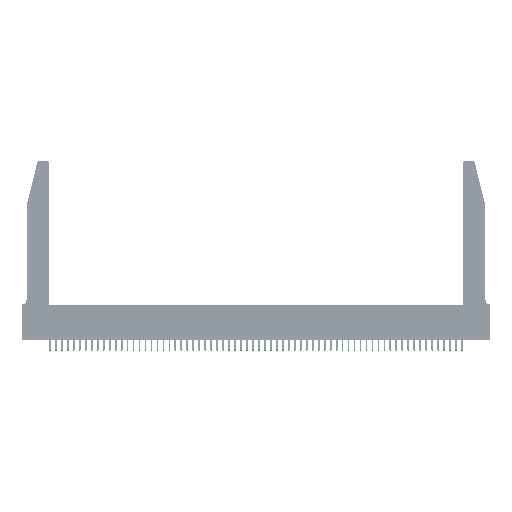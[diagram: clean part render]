
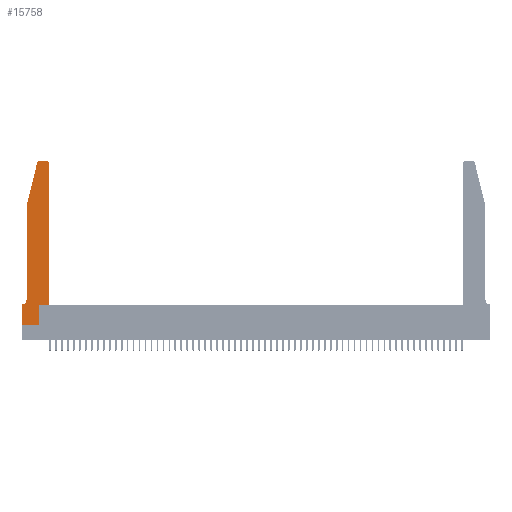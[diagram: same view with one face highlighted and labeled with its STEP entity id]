
A CAD part, top view. The second image highlights one B-rep face of the part: STEP entity #15758.
In plain terms, the highlighted planar face has unit normal (0, 0, 1).
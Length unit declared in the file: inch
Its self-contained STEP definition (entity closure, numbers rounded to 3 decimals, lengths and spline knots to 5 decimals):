
#101 = EDGE_CURVE ( 'NONE', #5792, #35913, #6823, .T. ) ;
#407 = VERTEX_POINT ( 'NONE', #45892 ) ;
#583 = LINE ( 'NONE', #42101, #45252 ) ;
#868 = VECTOR ( 'NONE', #31480, 39.37008 ) ;
#1223 = VERTEX_POINT ( 'NONE', #55118 ) ;
#1274 = EDGE_CURVE ( 'NONE', #35913, #38165, #583, .T. ) ;
#1558 = VECTOR ( 'NONE', #19152, 39.37008 ) ;
#2995 = DIRECTION ( 'NONE',  ( 0., 0., 1. ) ) ;
#3016 = DIRECTION ( 'NONE',  ( 0., 0., 1. ) ) ;
#3616 = CARTESIAN_POINT ( 'NONE',  ( 0., 0.35, 0.37 ) ) ;
#4064 = CARTESIAN_POINT ( 'NONE',  ( 0.0055, 0.35, 0.37 ) ) ;
#4310 = LINE ( 'NONE', #30976, #32062 ) ;
#5256 = EDGE_CURVE ( 'NONE', #407, #19347, #4310, .T. ) ;
#5743 = CARTESIAN_POINT ( 'NONE',  ( 0.4505, 0.35, 0.37 ) ) ;
#5792 = VERTEX_POINT ( 'NONE', #4064 ) ;
#6823 = LINE ( 'NONE', #33890, #46058 ) ;
#7276 = DIRECTION ( 'NONE',  ( 1., 0., 0. ) ) ;
#7305 = CARTESIAN_POINT ( 'NONE',  ( 0.0055, 0.42, 0.37 ) ) ;
#8950 = ORIENTED_EDGE ( 'NONE', *, *, #27693, .T. ) ;
#9331 = EDGE_LOOP ( 'NONE', ( #8950, #53865, #27278, #42686, #16671, #38875, #25576, #28283, #25086, #22221, #33995, #50335 ) ) ;
#10756 = EDGE_CURVE ( 'NONE', #41395, #11574, #15160, .T. ) ;
#11542 = DIRECTION ( 'NONE',  ( 0., 0., 1. ) ) ;
#11574 = VERTEX_POINT ( 'NONE', #22725 ) ;
#13098 = CARTESIAN_POINT ( 'NONE',  ( 0., 0., 0.37 ) ) ;
#15053 = CIRCLE ( 'NONE', #49882, 0.03 ) ;
#15160 = LINE ( 'NONE', #5743, #868 ) ;
#15224 = LINE ( 'NONE', #22927, #24682 ) ;
#15465 = AXIS2_PLACEMENT_3D ( 'NONE', #7305, #41891, #20745 ) ;
#15758 = ADVANCED_FACE ( 'NONE', ( #28016 ), #55628, .T. ) ;
#16457 = LINE ( 'NONE', #24059, #1558 ) ;
#16671 = ORIENTED_EDGE ( 'NONE', *, *, #50506, .T. ) ;
#17755 = CARTESIAN_POINT ( 'NONE',  ( 0.0755, 2., 0.37 ) ) ;
#19152 = DIRECTION ( 'NONE',  ( -1., 0., 0. ) ) ;
#19289 = EDGE_CURVE ( 'NONE', #19347, #20377, #46531, .T. ) ;
#19306 = DIRECTION ( 'NONE',  ( 0., 1., 0. ) ) ;
#19347 = VERTEX_POINT ( 'NONE', #17755 ) ;
#20377 = VERTEX_POINT ( 'NONE', #45859 ) ;
#20745 = DIRECTION ( 'NONE',  ( -1., 0., 0. ) ) ;
#20920 = LINE ( 'NONE', #24334, #43241 ) ;
#22221 = ORIENTED_EDGE ( 'NONE', *, *, #41916, .T. ) ;
#22725 = CARTESIAN_POINT ( 'NONE',  ( 0.4505, 2.72, 0.37 ) ) ;
#22927 = CARTESIAN_POINT ( 'NONE',  ( 0.2865, 0.35, 0.37 ) ) ;
#24059 = CARTESIAN_POINT ( 'NONE',  ( 0.2605, 2.75, 0.37 ) ) ;
#24334 = CARTESIAN_POINT ( 'NONE',  ( 0.4505, 0.35, 0.37 ) ) ;
#24589 = DIRECTION ( 'NONE',  ( 1., 0., 0. ) ) ;
#24682 = VECTOR ( 'NONE', #19306, 39.37008 ) ;
#25086 = ORIENTED_EDGE ( 'NONE', *, *, #36536, .T. ) ;
#25159 = CARTESIAN_POINT ( 'NONE',  ( 0.4505, 0.35, 0.37 ) ) ;
#25576 = ORIENTED_EDGE ( 'NONE', *, *, #1274, .T. ) ;
#25790 = DIRECTION ( 'NONE',  ( 1., 0., 0. ) ) ;
#26288 = AXIS2_PLACEMENT_3D ( 'NONE', #54805, #2995, #37589 ) ;
#26347 = LINE ( 'NONE', #13098, #45908 ) ;
#27278 = ORIENTED_EDGE ( 'NONE', *, *, #5256, .T. ) ;
#27693 = EDGE_CURVE ( 'NONE', #45223, #1223, #16457, .T. ) ;
#28016 = FACE_OUTER_BOUND ( 'NONE', #9331, .T. ) ;
#28283 = ORIENTED_EDGE ( 'NONE', *, *, #33462, .T. ) ;
#28641 = CARTESIAN_POINT ( 'NONE',  ( 0., 0., 0.37 ) ) ;
#30071 = CIRCLE ( 'NONE', #26288, 0.03 ) ;
#30976 = CARTESIAN_POINT ( 'NONE',  ( 0.0755, 2., 0.37 ) ) ;
#31480 = DIRECTION ( 'NONE',  ( 0., 1., 0. ) ) ;
#32062 = VECTOR ( 'NONE', #35497, 39.37008 ) ;
#33462 = EDGE_CURVE ( 'NONE', #38165, #39891, #26347, .T. ) ;
#33890 = CARTESIAN_POINT ( 'NONE',  ( 0.0755, 0.35, 0.37 ) ) ;
#33995 = ORIENTED_EDGE ( 'NONE', *, *, #10756, .T. ) ;
#34957 = CARTESIAN_POINT ( 'NONE',  ( 0.0755, 2., 0.37 ) ) ;
#35497 = DIRECTION ( 'NONE',  ( -0.239, -0.971, 0. ) ) ;
#35913 = VERTEX_POINT ( 'NONE', #53578 ) ;
#36536 = EDGE_CURVE ( 'NONE', #39891, #46829, #15224, .T. ) ;
#36779 = EDGE_CURVE ( 'NONE', #11574, #45223, #30071, .T. ) ;
#37046 = CARTESIAN_POINT ( 'NONE',  ( 0.284, 2.72, 0.37 ) ) ;
#37589 = DIRECTION ( 'NONE',  ( 1., 0., 0. ) ) ;
#37636 = CARTESIAN_POINT ( 'NONE',  ( 0.2865, 0.35, 0.37 ) ) ;
#37795 = EDGE_CURVE ( 'NONE', #1223, #407, #15053, .T. ) ;
#38165 = VERTEX_POINT ( 'NONE', #28641 ) ;
#38875 = ORIENTED_EDGE ( 'NONE', *, *, #101, .T. ) ;
#39060 = VECTOR ( 'NONE', #47475, 39.37008 ) ;
#39891 = VERTEX_POINT ( 'NONE', #47780 ) ;
#40790 = CARTESIAN_POINT ( 'NONE',  ( 0.4205, 2.75, 0.37 ) ) ;
#41395 = VERTEX_POINT ( 'NONE', #25159 ) ;
#41536 = DIRECTION ( 'NONE',  ( 0., -1., 0. ) ) ;
#41891 = DIRECTION ( 'NONE',  ( 0., 0., -1. ) ) ;
#41916 = EDGE_CURVE ( 'NONE', #46829, #41395, #20920, .T. ) ;
#41980 = DIRECTION ( 'NONE',  ( 1., 0., 0. ) ) ;
#42101 = CARTESIAN_POINT ( 'NONE',  ( 0., 0., 0.37 ) ) ;
#42686 = ORIENTED_EDGE ( 'NONE', *, *, #19289, .T. ) ;
#43241 = VECTOR ( 'NONE', #7276, 39.37008 ) ;
#43407 = AXIS2_PLACEMENT_3D ( 'NONE', #3616, #11542, #41980 ) ;
#45223 = VERTEX_POINT ( 'NONE', #40790 ) ;
#45252 = VECTOR ( 'NONE', #41536, 39.37008 ) ;
#45859 = CARTESIAN_POINT ( 'NONE',  ( 0.0755, 0.42, 0.37 ) ) ;
#45892 = CARTESIAN_POINT ( 'NONE',  ( 0.25487, 2.72718, 0.37 ) ) ;
#45908 = VECTOR ( 'NONE', #25790, 39.37008 ) ;
#46058 = VECTOR ( 'NONE', #51636, 39.37008 ) ;
#46531 = LINE ( 'NONE', #34957, #39060 ) ;
#46829 = VERTEX_POINT ( 'NONE', #37636 ) ;
#47475 = DIRECTION ( 'NONE',  ( 0., -1., 0. ) ) ;
#47780 = CARTESIAN_POINT ( 'NONE',  ( 0.2865, 0., 0.37 ) ) ;
#49882 = AXIS2_PLACEMENT_3D ( 'NONE', #37046, #3016, #24589 ) ;
#50244 = CIRCLE ( 'NONE', #15465, 0.07 ) ;
#50335 = ORIENTED_EDGE ( 'NONE', *, *, #36779, .T. ) ;
#50506 = EDGE_CURVE ( 'NONE', #20377, #5792, #50244, .T. ) ;
#51636 = DIRECTION ( 'NONE',  ( -1., 0., 0. ) ) ;
#53578 = CARTESIAN_POINT ( 'NONE',  ( 0., 0.35, 0.37 ) ) ;
#53865 = ORIENTED_EDGE ( 'NONE', *, *, #37795, .T. ) ;
#54805 = CARTESIAN_POINT ( 'NONE',  ( 0.4205, 2.72, 0.37 ) ) ;
#55118 = CARTESIAN_POINT ( 'NONE',  ( 0.284, 2.75, 0.37 ) ) ;
#55628 = PLANE ( 'NONE',  #43407 ) ;
